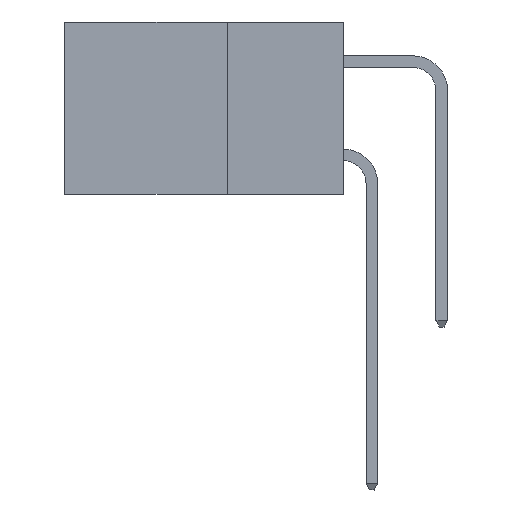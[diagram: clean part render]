
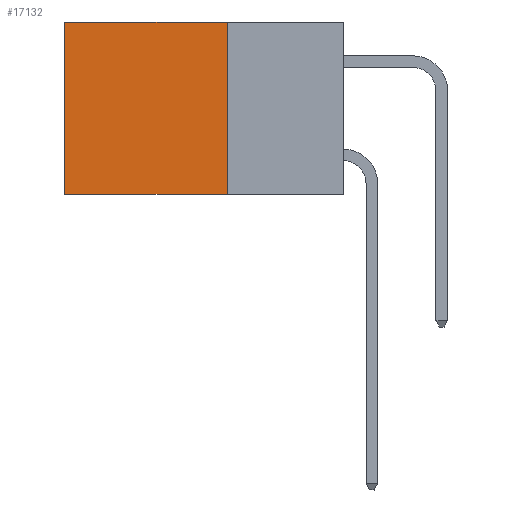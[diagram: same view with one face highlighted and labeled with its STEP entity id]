
A CAD part, left-side view. The second image highlights one B-rep face of the part: STEP entity #17132.
In plain terms, the highlighted planar face has unit normal (-1, 0, 0).
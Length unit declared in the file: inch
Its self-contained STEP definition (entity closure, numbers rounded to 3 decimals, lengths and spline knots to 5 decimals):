
#1102 = ORIENTED_EDGE ( 'NONE', *, *, #6647, .F. ) ;
#1741 = PLANE ( 'NONE',  #2993 ) ;
#2993 = AXIS2_PLACEMENT_3D ( 'NONE', #11092, #18728, #7218 ) ;
#6456 = EDGE_CURVE ( 'NONE', #8528, #10909, #18940, .T. ) ;
#6647 = EDGE_CURVE ( 'NONE', #10909, #7984, #12725, .T. ) ;
#6997 = CARTESIAN_POINT ( 'NONE',  ( 0.298, 0.25, -0.37 ) ) ;
#7218 = DIRECTION ( 'NONE',  ( 0., 0., -1. ) ) ;
#7680 = VECTOR ( 'NONE', #20264, 39.37008 ) ;
#7984 = VERTEX_POINT ( 'NONE', #11456 ) ;
#8055 = EDGE_CURVE ( 'NONE', #12032, #7984, #17387, .T. ) ;
#8093 = EDGE_CURVE ( 'NONE', #8528, #12032, #19441, .T. ) ;
#8528 = VERTEX_POINT ( 'NONE', #11992 ) ;
#9380 = VECTOR ( 'NONE', #22150, 39.37008 ) ;
#10535 = VECTOR ( 'NONE', #11733, 39.37008 ) ;
#10909 = VERTEX_POINT ( 'NONE', #22485 ) ;
#11092 = CARTESIAN_POINT ( 'NONE',  ( 0.298, 0.25, 0. ) ) ;
#11456 = CARTESIAN_POINT ( 'NONE',  ( 0.298, 0.6, -0.37 ) ) ;
#11733 = DIRECTION ( 'NONE',  ( 0., 1., 0. ) ) ;
#11992 = CARTESIAN_POINT ( 'NONE',  ( 0.298, 0.25, 0. ) ) ;
#12032 = VERTEX_POINT ( 'NONE', #24541 ) ;
#12109 = FACE_OUTER_BOUND ( 'NONE', #15808, .T. ) ;
#12725 = LINE ( 'NONE', #6997, #7680 ) ;
#13673 = CARTESIAN_POINT ( 'NONE',  ( 0.298, 0.25, 0. ) ) ;
#15808 = EDGE_LOOP ( 'NONE', ( #20339, #1102, #19471, #19355 ) ) ;
#17132 = ADVANCED_FACE ( 'NONE', ( #12109 ), #1741, .F. ) ;
#17387 = LINE ( 'NONE', #21740, #9380 ) ;
#17484 = VECTOR ( 'NONE', #24502, 39.37008 ) ;
#18728 = DIRECTION ( 'NONE',  ( 1., 0., 0. ) ) ;
#18940 = LINE ( 'NONE', #13673, #17484 ) ;
#19355 = ORIENTED_EDGE ( 'NONE', *, *, #8093, .T. ) ;
#19441 = LINE ( 'NONE', #21156, #10535 ) ;
#19471 = ORIENTED_EDGE ( 'NONE', *, *, #6456, .F. ) ;
#20264 = DIRECTION ( 'NONE',  ( 0., 1., 0. ) ) ;
#20339 = ORIENTED_EDGE ( 'NONE', *, *, #8055, .T. ) ;
#21156 = CARTESIAN_POINT ( 'NONE',  ( 0.298, 0.25, 0. ) ) ;
#21740 = CARTESIAN_POINT ( 'NONE',  ( 0.298, 0.6, 0. ) ) ;
#22150 = DIRECTION ( 'NONE',  ( 0., 0., -1. ) ) ;
#22485 = CARTESIAN_POINT ( 'NONE',  ( 0.298, 0.25, -0.37 ) ) ;
#24502 = DIRECTION ( 'NONE',  ( 0., 0., -1. ) ) ;
#24541 = CARTESIAN_POINT ( 'NONE',  ( 0.298, 0.6, 0. ) ) ;
